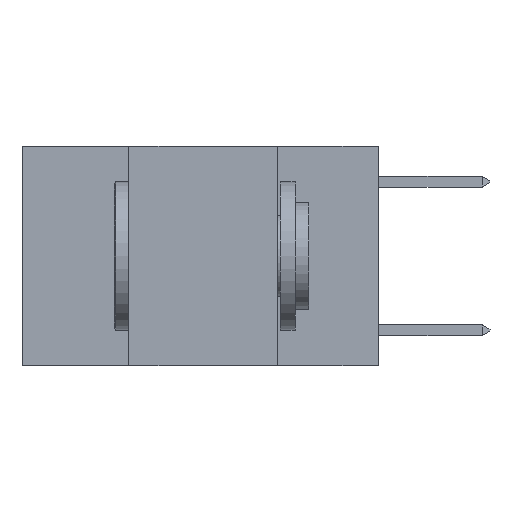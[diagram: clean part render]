
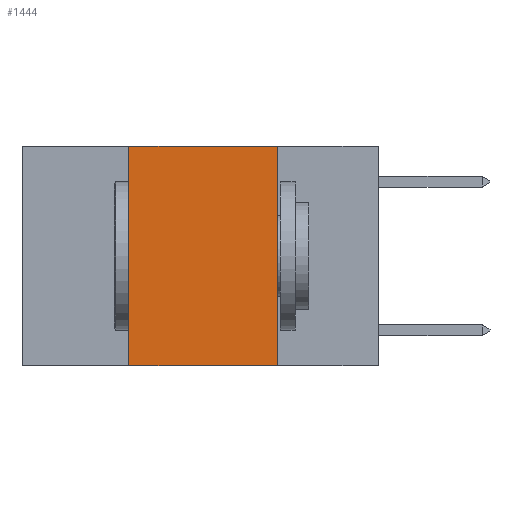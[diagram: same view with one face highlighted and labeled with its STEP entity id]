
A CAD part, left-side view. The second image highlights one B-rep face of the part: STEP entity #1444.
In plain terms, the highlighted planar face has unit normal (-1, 0, 0).
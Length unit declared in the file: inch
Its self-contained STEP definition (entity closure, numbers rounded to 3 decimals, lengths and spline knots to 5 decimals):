
#516 = EDGE_CURVE ( 'NONE', #5934, #4116, #2962, .T. ) ;
#883 = DIRECTION ( 'NONE',  ( 0., -1., 0. ) ) ;
#1016 = ORIENTED_EDGE ( 'NONE', *, *, #7225, .F. ) ;
#1110 = DIRECTION ( 'NONE',  ( 0., -1., 0. ) ) ;
#1444 = ADVANCED_FACE ( 'NONE', ( #2379 ), #6981, .F. ) ;
#1453 = EDGE_LOOP ( 'NONE', ( #3474, #7749, #1016, #3978 ) ) ;
#1531 = CARTESIAN_POINT ( 'NONE',  ( 0., 0.17, 0. ) ) ;
#1783 = LINE ( 'NONE', #7813, #4612 ) ;
#2220 = LINE ( 'NONE', #10920, #11390 ) ;
#2379 = FACE_OUTER_BOUND ( 'NONE', #1453, .T. ) ;
#2579 = DIRECTION ( 'NONE',  ( 0., 0., -1. ) ) ;
#2962 = LINE ( 'NONE', #8377, #10062 ) ;
#3474 = ORIENTED_EDGE ( 'NONE', *, *, #5542, .F. ) ;
#3978 = ORIENTED_EDGE ( 'NONE', *, *, #516, .T. ) ;
#4116 = VERTEX_POINT ( 'NONE', #4740 ) ;
#4168 = VECTOR ( 'NONE', #2579, 39.37008 ) ;
#4566 = CARTESIAN_POINT ( 'NONE',  ( 0., 0.42, 0. ) ) ;
#4612 = VECTOR ( 'NONE', #8663, 39.37008 ) ;
#4709 = AXIS2_PLACEMENT_3D ( 'NONE', #7603, #6842, #4824 ) ;
#4740 = CARTESIAN_POINT ( 'NONE',  ( 0., 0.17, -0.37 ) ) ;
#4824 = DIRECTION ( 'NONE',  ( 0., 0., -1. ) ) ;
#5476 = VERTEX_POINT ( 'NONE', #1531 ) ;
#5542 = EDGE_CURVE ( 'NONE', #5476, #4116, #6508, .T. ) ;
#5934 = VERTEX_POINT ( 'NONE', #6578 ) ;
#6508 = LINE ( 'NONE', #7951, #4168 ) ;
#6526 = VERTEX_POINT ( 'NONE', #4566 ) ;
#6578 = CARTESIAN_POINT ( 'NONE',  ( 0., 0.42, -0.37 ) ) ;
#6842 = DIRECTION ( 'NONE',  ( 1., 0., 0. ) ) ;
#6920 = EDGE_CURVE ( 'NONE', #6526, #5476, #2220, .T. ) ;
#6981 = PLANE ( 'NONE',  #4709 ) ;
#7225 = EDGE_CURVE ( 'NONE', #5934, #6526, #1783, .T. ) ;
#7603 = CARTESIAN_POINT ( 'NONE',  ( 0., 0.6, 0. ) ) ;
#7749 = ORIENTED_EDGE ( 'NONE', *, *, #6920, .F. ) ;
#7813 = CARTESIAN_POINT ( 'NONE',  ( 0., 0.42, 0. ) ) ;
#7951 = CARTESIAN_POINT ( 'NONE',  ( 0., 0.17, 0. ) ) ;
#8377 = CARTESIAN_POINT ( 'NONE',  ( 0., 0.6, -0.37 ) ) ;
#8663 = DIRECTION ( 'NONE',  ( 0., 0., 1. ) ) ;
#10062 = VECTOR ( 'NONE', #883, 39.37008 ) ;
#10920 = CARTESIAN_POINT ( 'NONE',  ( 0., 0.6, 0. ) ) ;
#11390 = VECTOR ( 'NONE', #1110, 39.37008 ) ;
